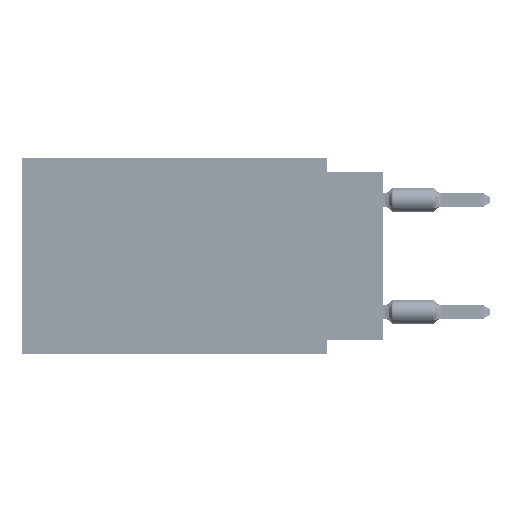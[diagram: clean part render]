
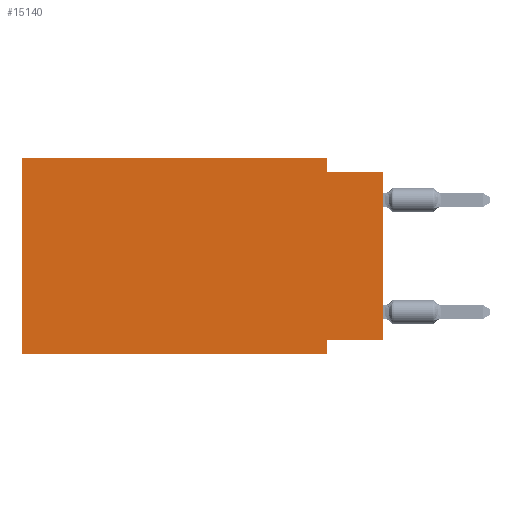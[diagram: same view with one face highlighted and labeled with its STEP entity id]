
A CAD part, left-side view. The second image highlights one B-rep face of the part: STEP entity #15140.
In plain terms, the highlighted planar face has unit normal (-1, 0, 0).
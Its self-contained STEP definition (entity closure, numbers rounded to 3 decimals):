
#433 = ORIENTED_EDGE ( 'NONE', *, *, #89317, .T. ) ;
#1435 = CARTESIAN_POINT ( 'NONE',  ( 0., 16.383, 0. ) ) ;
#1846 = LINE ( 'NONE', #47651, #11529 ) ;
#2091 = DIRECTION ( 'NONE',  ( 0., 0., -1. ) ) ;
#3883 = EDGE_CURVE ( 'NONE', #52820, #90428, #68390, .T. ) ;
#5542 = CARTESIAN_POINT ( 'NONE',  ( 0., 2.54, 0. ) ) ;
#7508 = CARTESIAN_POINT ( 'NONE',  ( 0., 2.54, -8.89 ) ) ;
#7569 = ORIENTED_EDGE ( 'NONE', *, *, #30473, .F. ) ;
#7673 = DIRECTION ( 'NONE',  ( 0., 0., -1. ) ) ;
#10022 = LINE ( 'NONE', #66063, #60317 ) ;
#11529 = VECTOR ( 'NONE', #63590, 1000. ) ;
#15140 = ADVANCED_FACE ( 'NONE', ( #24268 ), #87973, .F. ) ;
#15226 = DIRECTION ( 'NONE',  ( 0., 0., -1. ) ) ;
#15378 = CARTESIAN_POINT ( 'NONE',  ( 0., 2.54, 0. ) ) ;
#15992 = EDGE_LOOP ( 'NONE', ( #87565, #44043, #90529, #7569, #71132, #433, #27309, #60288 ) ) ;
#16355 = LINE ( 'NONE', #1435, #96486 ) ;
#17549 = CARTESIAN_POINT ( 'NONE',  ( 0., 16.383, 0. ) ) ;
#19778 = CARTESIAN_POINT ( 'NONE',  ( 0., 16.383, 0. ) ) ;
#20669 = VERTEX_POINT ( 'NONE', #57716 ) ;
#21833 = LINE ( 'NONE', #53727, #24780 ) ;
#21884 = VERTEX_POINT ( 'NONE', #36113 ) ;
#24268 = FACE_OUTER_BOUND ( 'NONE', #15992, .T. ) ;
#24727 = LINE ( 'NONE', #57600, #50758 ) ;
#24780 = VECTOR ( 'NONE', #37782, 1000. ) ;
#27309 = ORIENTED_EDGE ( 'NONE', *, *, #73755, .F. ) ;
#28230 = VERTEX_POINT ( 'NONE', #37617 ) ;
#29626 = LINE ( 'NONE', #85149, #50885 ) ;
#30111 = DIRECTION ( 'NONE',  ( 0., 0., 1. ) ) ;
#30473 = EDGE_CURVE ( 'NONE', #97632, #52820, #1846, .T. ) ;
#36113 = CARTESIAN_POINT ( 'NONE',  ( 0., 0., -8.255 ) ) ;
#36720 = CARTESIAN_POINT ( 'NONE',  ( 0., 2.54, -0.635 ) ) ;
#37611 = VECTOR ( 'NONE', #15226, 1000. ) ;
#37617 = CARTESIAN_POINT ( 'NONE',  ( 0., 0., -0.635 ) ) ;
#37782 = DIRECTION ( 'NONE',  ( 0., -1., 0. ) ) ;
#44043 = ORIENTED_EDGE ( 'NONE', *, *, #75392, .F. ) ;
#47651 = CARTESIAN_POINT ( 'NONE',  ( 0., 16.383, 0. ) ) ;
#48008 = EDGE_CURVE ( 'NONE', #74189, #97632, #16355, .T. ) ;
#48726 = DIRECTION ( 'NONE',  ( 0., 0., 1. ) ) ;
#48909 = DIRECTION ( 'NONE',  ( 1., 0., 0. ) ) ;
#49367 = DIRECTION ( 'NONE',  ( 0., -1., 0. ) ) ;
#50758 = VECTOR ( 'NONE', #49367, 1000. ) ;
#50885 = VECTOR ( 'NONE', #30111, 1000. ) ;
#52820 = VERTEX_POINT ( 'NONE', #5542 ) ;
#53430 = EDGE_CURVE ( 'NONE', #21884, #28230, #29626, .T. ) ;
#53727 = CARTESIAN_POINT ( 'NONE',  ( 0., 0., -0.635 ) ) ;
#57017 = VECTOR ( 'NONE', #7673, 1000. ) ;
#57600 = CARTESIAN_POINT ( 'NONE',  ( 0., 16.383, -8.89 ) ) ;
#57716 = CARTESIAN_POINT ( 'NONE',  ( 0., 2.54, -8.89 ) ) ;
#60288 = ORIENTED_EDGE ( 'NONE', *, *, #63110, .F. ) ;
#60317 = VECTOR ( 'NONE', #82018, 1000. ) ;
#63110 = EDGE_CURVE ( 'NONE', #21884, #65180, #10022, .T. ) ;
#63590 = DIRECTION ( 'NONE',  ( 0., -1., 0. ) ) ;
#65180 = VERTEX_POINT ( 'NONE', #84733 ) ;
#66063 = CARTESIAN_POINT ( 'NONE',  ( 0., 0., -8.255 ) ) ;
#68390 = LINE ( 'NONE', #15378, #57017 ) ;
#71132 = ORIENTED_EDGE ( 'NONE', *, *, #48008, .F. ) ;
#73755 = EDGE_CURVE ( 'NONE', #65180, #20669, #91889, .T. ) ;
#74189 = VERTEX_POINT ( 'NONE', #86980 ) ;
#75392 = EDGE_CURVE ( 'NONE', #90428, #28230, #21833, .T. ) ;
#82018 = DIRECTION ( 'NONE',  ( 0., 1., 0. ) ) ;
#82928 = AXIS2_PLACEMENT_3D ( 'NONE', #17549, #48909, #2091 ) ;
#84733 = CARTESIAN_POINT ( 'NONE',  ( 0., 2.54, -8.255 ) ) ;
#85149 = CARTESIAN_POINT ( 'NONE',  ( 0., 0., 0. ) ) ;
#86980 = CARTESIAN_POINT ( 'NONE',  ( 0., 16.383, -8.89 ) ) ;
#87565 = ORIENTED_EDGE ( 'NONE', *, *, #53430, .T. ) ;
#87973 = PLANE ( 'NONE',  #82928 ) ;
#89317 = EDGE_CURVE ( 'NONE', #74189, #20669, #24727, .T. ) ;
#90428 = VERTEX_POINT ( 'NONE', #36720 ) ;
#90529 = ORIENTED_EDGE ( 'NONE', *, *, #3883, .F. ) ;
#91889 = LINE ( 'NONE', #7508, #37611 ) ;
#96486 = VECTOR ( 'NONE', #48726, 1000. ) ;
#97632 = VERTEX_POINT ( 'NONE', #19778 ) ;
